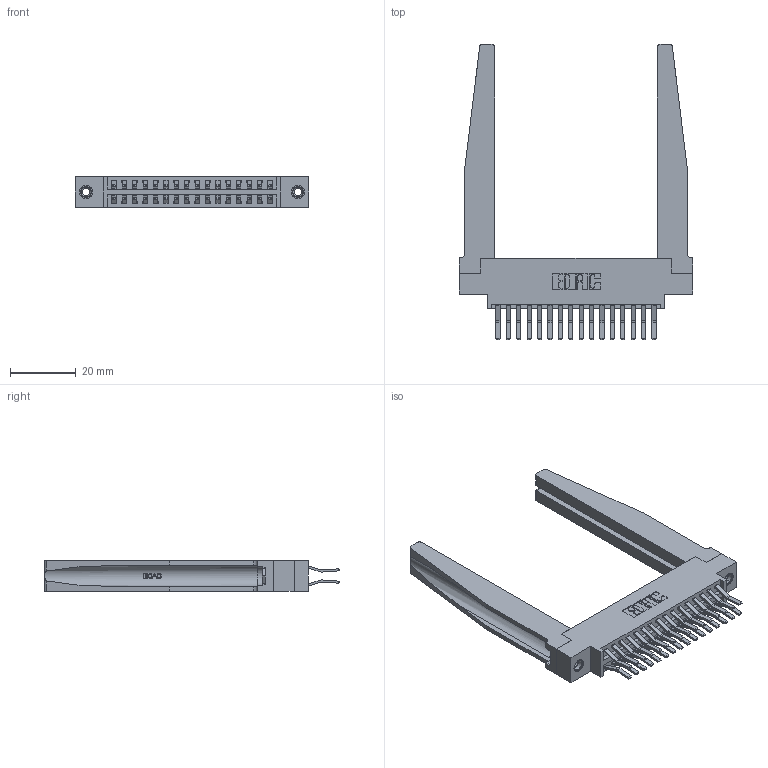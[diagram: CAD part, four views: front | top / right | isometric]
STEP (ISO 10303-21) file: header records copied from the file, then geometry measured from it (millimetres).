
FILE_DESCRIPTION (( 'STEP AP203' ), '1' );
FILE_NAME ('396-032-560-878.STEP', '2019-11-01T20:13:01', ( '' ), ( '' ), 'SwSTEP 2.0', 'SolidWorks 2016', '' );
FILE_SCHEMA (( 'CONFIG_CONTROL_DESIGN' ));
Length unit declared in the file: inch
Products named in the file (5): 396-032-560-878; 346 Part_0.170 Offset - 0.156 Dia-TH; 345-292-001_560 Tail; 346-220-078_345-220-078; 345-250-001_345-250-001-102
Assembly tree (37 placements, depth 2):
  396-032-560-878
    346 Part_0.170 Offset - 0.156 Dia-TH
    345-292-001_560 Tail  x32
    346-220-078_345-220-078  x2
    345-250-001_345-250-001-102  x2
Bounding box: 71.37 x 90.05 x 9.4 mm (x, y, z)
Volume: 13721.9 mm3; surface area: 16233.1 mm2
Topology: 37 solids, 37 shells, 2088 faces, 6101 edges, 4014 vertices
Faces by surface type: plane 1342, cylinder 694, bspline 36, cone 12, torus 4
Entity records: 18910 total; most frequent: CARTESIAN_POINT 4091, ORIENTED_EDGE 2914, DIRECTION 2647, EDGE_CURVE 1457, VECTOR 1163, LINE 1163, VERTEX_POINT 964, AXIS2_PLACEMENT_3D 742
